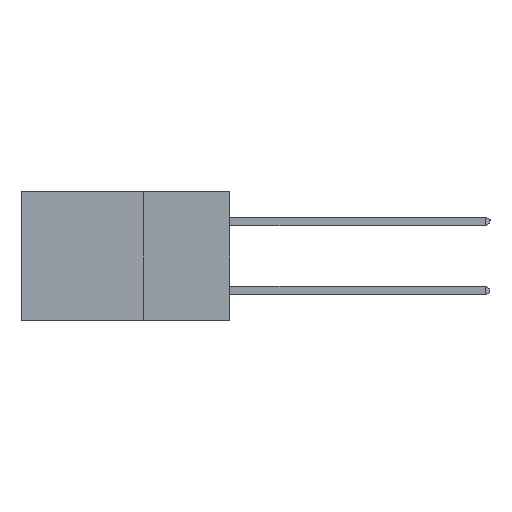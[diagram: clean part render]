
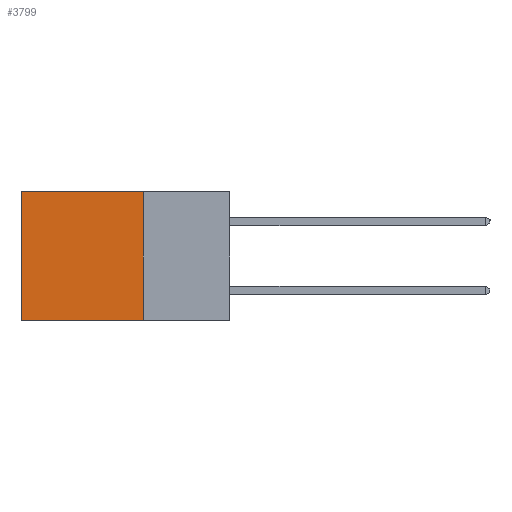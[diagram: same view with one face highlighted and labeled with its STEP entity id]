
A CAD part, left-side view. The second image highlights one B-rep face of the part: STEP entity #3799.
In plain terms, the highlighted planar face has unit normal (-1, 0, 0).
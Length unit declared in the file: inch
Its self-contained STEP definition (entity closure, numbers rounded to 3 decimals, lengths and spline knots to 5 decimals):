
#829 = VERTEX_POINT ( 'NONE', #10645 ) ;
#2314 = ORIENTED_EDGE ( 'NONE', *, *, #2430, .F. ) ;
#2379 = ORIENTED_EDGE ( 'NONE', *, *, #7268, .T. ) ;
#2430 = EDGE_CURVE ( 'NONE', #9152, #6411, #3649, .T. ) ;
#2882 = EDGE_CURVE ( 'NONE', #12101, #6411, #8037, .T. ) ;
#3206 = PLANE ( 'NONE',  #11363 ) ;
#3482 = VECTOR ( 'NONE', #13843, 39.37008 ) ;
#3649 = LINE ( 'NONE', #8129, #13780 ) ;
#3799 = ADVANCED_FACE ( 'NONE', ( #14225 ), #3206, .F. ) ;
#3979 = LINE ( 'NONE', #6310, #7059 ) ;
#4154 = CARTESIAN_POINT ( 'NONE',  ( 0.2615, 0.25, -0.37 ) ) ;
#4817 = DIRECTION ( 'NONE',  ( 0., 1., 0. ) ) ;
#4979 = DIRECTION ( 'NONE',  ( 0., 0., -1. ) ) ;
#5439 = VECTOR ( 'NONE', #10959, 39.37008 ) ;
#5526 = CARTESIAN_POINT ( 'NONE',  ( 0.2615, 0.6, 0. ) ) ;
#5563 = CARTESIAN_POINT ( 'NONE',  ( 0.2615, 0.25, -0.37 ) ) ;
#6310 = CARTESIAN_POINT ( 'NONE',  ( 0.2615, 0.25, 0. ) ) ;
#6411 = VERTEX_POINT ( 'NONE', #7311 ) ;
#7033 = ORIENTED_EDGE ( 'NONE', *, *, #2882, .T. ) ;
#7059 = VECTOR ( 'NONE', #8310, 39.37008 ) ;
#7268 = EDGE_CURVE ( 'NONE', #829, #12101, #3979, .T. ) ;
#7311 = CARTESIAN_POINT ( 'NONE',  ( 0.2615, 0.6, -0.37 ) ) ;
#8037 = LINE ( 'NONE', #9283, #3482 ) ;
#8129 = CARTESIAN_POINT ( 'NONE',  ( 0.2615, 0.25, -0.37 ) ) ;
#8310 = DIRECTION ( 'NONE',  ( 0., 1., 0. ) ) ;
#8677 = LINE ( 'NONE', #13170, #5439 ) ;
#9111 = EDGE_LOOP ( 'NONE', ( #7033, #2314, #9737, #2379 ) ) ;
#9152 = VERTEX_POINT ( 'NONE', #5563 ) ;
#9283 = CARTESIAN_POINT ( 'NONE',  ( 0.2615, 0.6, -0.37 ) ) ;
#9737 = ORIENTED_EDGE ( 'NONE', *, *, #10004, .F. ) ;
#10004 = EDGE_CURVE ( 'NONE', #829, #9152, #8677, .T. ) ;
#10645 = CARTESIAN_POINT ( 'NONE',  ( 0.2615, 0.25, 0. ) ) ;
#10959 = DIRECTION ( 'NONE',  ( 0., 0., -1. ) ) ;
#11363 = AXIS2_PLACEMENT_3D ( 'NONE', #4154, #11678, #4979 ) ;
#11678 = DIRECTION ( 'NONE',  ( 1., 0., 0. ) ) ;
#12101 = VERTEX_POINT ( 'NONE', #5526 ) ;
#13170 = CARTESIAN_POINT ( 'NONE',  ( 0.2615, 0.25, -0.37 ) ) ;
#13780 = VECTOR ( 'NONE', #4817, 39.37008 ) ;
#13843 = DIRECTION ( 'NONE',  ( 0., 0., -1. ) ) ;
#14225 = FACE_OUTER_BOUND ( 'NONE', #9111, .T. ) ;
